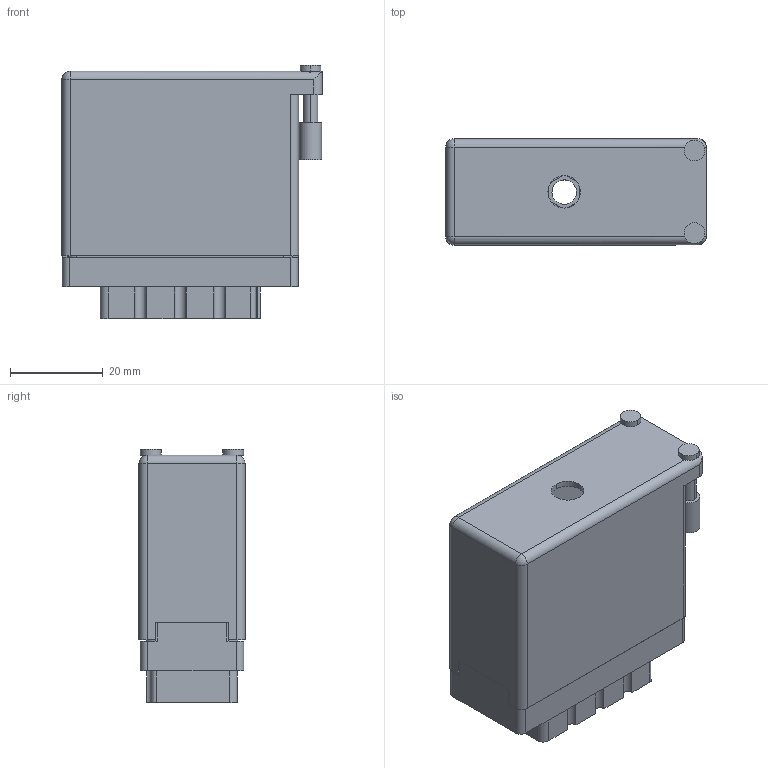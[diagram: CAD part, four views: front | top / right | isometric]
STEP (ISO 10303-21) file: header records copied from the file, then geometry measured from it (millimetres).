
FILE_DESCRIPTION (( 'STEP AP203' ), '1' );
FILE_NAME ('516-038-520-250.STEP', '2020-03-05T13:21:43', ( '' ), ( '' ), 'SwSTEP 2.0', 'SolidWorks 2016', '' );
FILE_SCHEMA (( 'CONFIG_CONTROL_DESIGN' ));
Length unit declared in the file: inch
Products named in the file (4): 516-230-001_Metal - 038 Side Entry; 516 Part Receptacle_038; 516-038-520-250; 516-292-001_520 Contact
Assembly tree (40 placements, depth 2):
  516-038-520-250
    516 Part Receptacle_038
    516-292-001_520 Contact  x38
    516-230-001_Metal - 038 Side Entry
Bounding box: 56.08 x 22.83 x 54.53 mm (x, y, z)
Volume: 20672.9 mm3; surface area: 34280.7 mm2
Topology: 40 solids, 40 shells, 3715 faces, 10767 edges, 7146 vertices
Faces by surface type: plane 2266, cylinder 1217, bspline 228, cone 2, sphere 2
Entity records: 36841 total; most frequent: CARTESIAN_POINT 6529, ORIENTED_EDGE 6138, DIRECTION 6006, EDGE_CURVE 3069, VECTOR 2230, LINE 2230, VERTEX_POINT 2040, AXIS2_PLACEMENT_3D 1888
